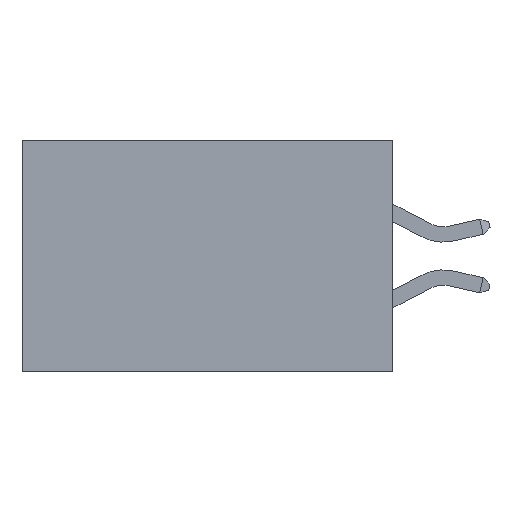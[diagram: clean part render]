
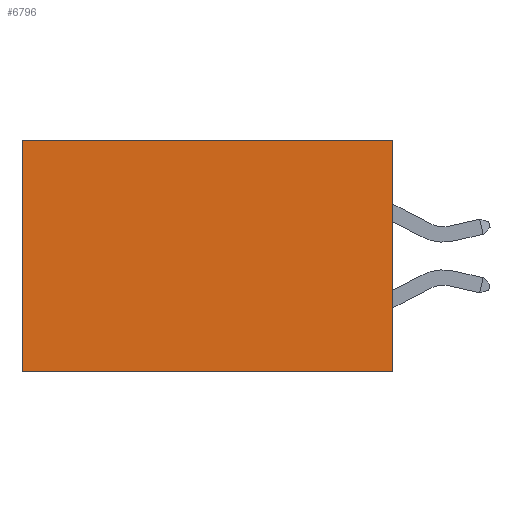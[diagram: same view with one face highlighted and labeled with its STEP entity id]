
A CAD part, left-side view. The second image highlights one B-rep face of the part: STEP entity #6796.
In plain terms, the highlighted planar face has unit normal (-1, 0, 0).
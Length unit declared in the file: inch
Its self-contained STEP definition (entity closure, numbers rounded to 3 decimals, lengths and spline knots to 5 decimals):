
#257 = VECTOR ( 'NONE', #4429, 39.37008 ) ;
#322 = VERTEX_POINT ( 'NONE', #2883 ) ;
#2022 = CARTESIAN_POINT ( 'NONE',  ( 0.2875, 0., -0.375 ) ) ;
#2883 = CARTESIAN_POINT ( 'NONE',  ( 0.2875, 0.6, 0. ) ) ;
#2957 = DIRECTION ( 'NONE',  ( 0., 1., 0. ) ) ;
#3503 = CARTESIAN_POINT ( 'NONE',  ( 0.2875, 0., -0.375 ) ) ;
#4252 = CARTESIAN_POINT ( 'NONE',  ( 0.2875, 0.6, -0.375 ) ) ;
#4404 = LINE ( 'NONE', #2022, #257 ) ;
#4429 = DIRECTION ( 'NONE',  ( 0., 0., -1. ) ) ;
#4616 = PLANE ( 'NONE',  #7659 ) ;
#5139 = LINE ( 'NONE', #10143, #15562 ) ;
#5160 = EDGE_CURVE ( 'NONE', #11172, #322, #5139, .T. ) ;
#5751 = ORIENTED_EDGE ( 'NONE', *, *, #9617, .F. ) ;
#6796 = ADVANCED_FACE ( 'NONE', ( #11473 ), #4616, .F. ) ;
#7194 = DIRECTION ( 'NONE',  ( 0., 0., -1. ) ) ;
#7270 = VERTEX_POINT ( 'NONE', #10198 ) ;
#7659 = AXIS2_PLACEMENT_3D ( 'NONE', #3503, #8191, #7194 ) ;
#8191 = DIRECTION ( 'NONE',  ( 1., 0., 0. ) ) ;
#8508 = CARTESIAN_POINT ( 'NONE',  ( 0.2875, 0., -0.375 ) ) ;
#8590 = EDGE_CURVE ( 'NONE', #13569, #7270, #10874, .T. ) ;
#9418 = EDGE_LOOP ( 'NONE', ( #10559, #14236, #5751, #14375 ) ) ;
#9617 = EDGE_CURVE ( 'NONE', #11172, #13569, #4404, .T. ) ;
#10143 = CARTESIAN_POINT ( 'NONE',  ( 0.2875, 0., 0. ) ) ;
#10198 = CARTESIAN_POINT ( 'NONE',  ( 0.2875, 0.6, -0.375 ) ) ;
#10491 = VECTOR ( 'NONE', #15588, 39.37008 ) ;
#10559 = ORIENTED_EDGE ( 'NONE', *, *, #14184, .T. ) ;
#10699 = LINE ( 'NONE', #4252, #13551 ) ;
#10874 = LINE ( 'NONE', #8508, #10491 ) ;
#11172 = VERTEX_POINT ( 'NONE', #14131 ) ;
#11473 = FACE_OUTER_BOUND ( 'NONE', #9418, .T. ) ;
#11942 = DIRECTION ( 'NONE',  ( 0., 0., -1. ) ) ;
#12134 = CARTESIAN_POINT ( 'NONE',  ( 0.2875, 0., -0.375 ) ) ;
#13551 = VECTOR ( 'NONE', #11942, 39.37008 ) ;
#13569 = VERTEX_POINT ( 'NONE', #12134 ) ;
#14131 = CARTESIAN_POINT ( 'NONE',  ( 0.2875, 0., 0. ) ) ;
#14184 = EDGE_CURVE ( 'NONE', #322, #7270, #10699, .T. ) ;
#14236 = ORIENTED_EDGE ( 'NONE', *, *, #8590, .F. ) ;
#14375 = ORIENTED_EDGE ( 'NONE', *, *, #5160, .T. ) ;
#15562 = VECTOR ( 'NONE', #2957, 39.37008 ) ;
#15588 = DIRECTION ( 'NONE',  ( 0., 1., 0. ) ) ;
